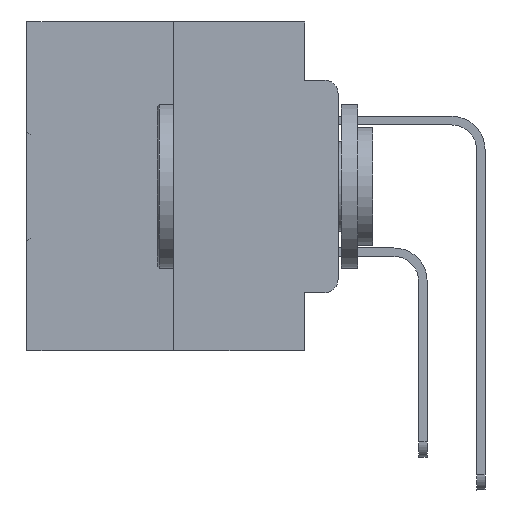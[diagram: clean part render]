
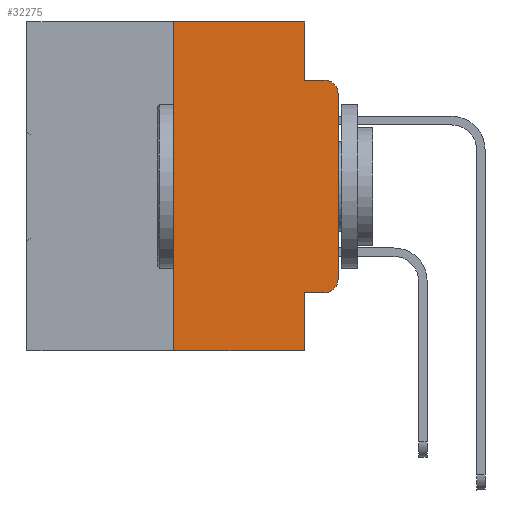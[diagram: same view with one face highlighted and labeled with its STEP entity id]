
A CAD part, left-side view. The second image highlights one B-rep face of the part: STEP entity #32275.
In plain terms, the highlighted planar face has unit normal (-1, 0, 0).
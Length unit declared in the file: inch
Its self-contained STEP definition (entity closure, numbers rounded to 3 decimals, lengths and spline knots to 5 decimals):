
#17 = ORIENTED_EDGE ( 'NONE', *, *, #22693, .F. ) ;
#160 = CARTESIAN_POINT ( 'NONE',  ( 0., 0.25, -0.5 ) ) ;
#294 = VERTEX_POINT ( 'NONE', #9027 ) ;
#494 = CARTESIAN_POINT ( 'NONE',  ( 0., 0.051, 0. ) ) ;
#1217 = VERTEX_POINT ( 'NONE', #7982 ) ;
#1354 = EDGE_LOOP ( 'NONE', ( #4849, #23765, #13144, #14403, #23952, #17, #20782, #31166, #22325, #22549 ) ) ;
#1962 = EDGE_CURVE ( 'NONE', #12531, #294, #4394, .T. ) ;
#2520 = DIRECTION ( 'NONE',  ( 0., 0., -1. ) ) ;
#3764 = DIRECTION ( 'NONE',  ( 0., -1., 0. ) ) ;
#4275 = AXIS2_PLACEMENT_3D ( 'NONE', #15778, #12622, #2520 ) ;
#4394 = LINE ( 'NONE', #23625, #15145 ) ;
#4592 = CARTESIAN_POINT ( 'NONE',  ( 0., 0.02, -0.1085 ) ) ;
#4849 = ORIENTED_EDGE ( 'NONE', *, *, #17953, .T. ) ;
#4910 = LINE ( 'NONE', #23252, #16567 ) ;
#6462 = VERTEX_POINT ( 'NONE', #9750 ) ;
#6599 = VERTEX_POINT ( 'NONE', #13415 ) ;
#6658 = LINE ( 'NONE', #19601, #23281 ) ;
#7982 = CARTESIAN_POINT ( 'NONE',  ( 0., 0.02, -0.0885 ) ) ;
#8341 = AXIS2_PLACEMENT_3D ( 'NONE', #23910, #29154, #18485 ) ;
#8583 = VERTEX_POINT ( 'NONE', #11410 ) ;
#8938 = DIRECTION ( 'NONE',  ( 0., 0., 1. ) ) ;
#9027 = CARTESIAN_POINT ( 'NONE',  ( 0., 0.051, -0.0885 ) ) ;
#9750 = CARTESIAN_POINT ( 'NONE',  ( 0., 0., -0.1085 ) ) ;
#10086 = EDGE_CURVE ( 'NONE', #6462, #1217, #32344, .T. ) ;
#10628 = VECTOR ( 'NONE', #26428, 39.37008 ) ;
#11410 = CARTESIAN_POINT ( 'NONE',  ( 0., 0.051, -0.4115 ) ) ;
#11671 = VECTOR ( 'NONE', #28363, 39.37008 ) ;
#11868 = VERTEX_POINT ( 'NONE', #20159 ) ;
#11936 = CARTESIAN_POINT ( 'NONE',  ( 0., 0., 0. ) ) ;
#12411 = DIRECTION ( 'NONE',  ( 0., 0., -1. ) ) ;
#12504 = VERTEX_POINT ( 'NONE', #160 ) ;
#12531 = VERTEX_POINT ( 'NONE', #494 ) ;
#12622 = DIRECTION ( 'NONE',  ( -1., 0., 0. ) ) ;
#13144 = ORIENTED_EDGE ( 'NONE', *, *, #33057, .F. ) ;
#13415 = CARTESIAN_POINT ( 'NONE',  ( 0., 0.25, 0. ) ) ;
#14403 = ORIENTED_EDGE ( 'NONE', *, *, #1962, .F. ) ;
#15058 = DIRECTION ( 'NONE',  ( 0., 0., 1. ) ) ;
#15145 = VECTOR ( 'NONE', #26060, 39.37008 ) ;
#15373 = CARTESIAN_POINT ( 'NONE',  ( 0., 0.473, -0.5 ) ) ;
#15761 = CARTESIAN_POINT ( 'NONE',  ( 0., 0.051, -0.0885 ) ) ;
#15778 = CARTESIAN_POINT ( 'NONE',  ( 0., 0.02, -0.3915 ) ) ;
#15942 = CARTESIAN_POINT ( 'NONE',  ( 0., 0.051, -0.5 ) ) ;
#16567 = VECTOR ( 'NONE', #12411, 39.37008 ) ;
#17953 = EDGE_CURVE ( 'NONE', #22711, #6462, #28353, .T. ) ;
#18129 = EDGE_CURVE ( 'NONE', #11868, #22711, #21593, .T. ) ;
#18485 = DIRECTION ( 'NONE',  ( 0., 0., -1. ) ) ;
#18568 = EDGE_CURVE ( 'NONE', #8583, #31263, #4910, .T. ) ;
#18815 = FACE_OUTER_BOUND ( 'NONE', #1354, .T. ) ;
#18874 = LINE ( 'NONE', #15373, #27511 ) ;
#19424 = CARTESIAN_POINT ( 'NONE',  ( 0., 0., -0.3915 ) ) ;
#19601 = CARTESIAN_POINT ( 'NONE',  ( 0., 0.25, 0. ) ) ;
#19784 = VECTOR ( 'NONE', #3764, 39.37008 ) ;
#20159 = CARTESIAN_POINT ( 'NONE',  ( 0., 0.02, -0.4115 ) ) ;
#20326 = LINE ( 'NONE', #28724, #11671 ) ;
#20782 = ORIENTED_EDGE ( 'NONE', *, *, #24681, .T. ) ;
#21019 = LINE ( 'NONE', #15761, #10628 ) ;
#21111 = PLANE ( 'NONE',  #8341 ) ;
#21593 = CIRCLE ( 'NONE', #4275, 0.02 ) ;
#22325 = ORIENTED_EDGE ( 'NONE', *, *, #32499, .T. ) ;
#22549 = ORIENTED_EDGE ( 'NONE', *, *, #18129, .T. ) ;
#22693 = EDGE_CURVE ( 'NONE', #12504, #6599, #6658, .T. ) ;
#22711 = VERTEX_POINT ( 'NONE', #19424 ) ;
#23252 = CARTESIAN_POINT ( 'NONE',  ( 0., 0.051, 0. ) ) ;
#23281 = VECTOR ( 'NONE', #8938, 39.37008 ) ;
#23625 = CARTESIAN_POINT ( 'NONE',  ( 0., 0.051, 0. ) ) ;
#23765 = ORIENTED_EDGE ( 'NONE', *, *, #10086, .T. ) ;
#23910 = CARTESIAN_POINT ( 'NONE',  ( 0., 0.473, 0. ) ) ;
#23952 = ORIENTED_EDGE ( 'NONE', *, *, #27161, .F. ) ;
#24681 = EDGE_CURVE ( 'NONE', #12504, #31263, #18874, .T. ) ;
#26051 = DIRECTION ( 'NONE',  ( 0., -1., 0. ) ) ;
#26060 = DIRECTION ( 'NONE',  ( 0., 0., -1. ) ) ;
#26185 = AXIS2_PLACEMENT_3D ( 'NONE', #4592, #31144, #27819 ) ;
#26428 = DIRECTION ( 'NONE',  ( 0., -1., 0. ) ) ;
#26591 = VECTOR ( 'NONE', #15058, 39.37008 ) ;
#27161 = EDGE_CURVE ( 'NONE', #6599, #12531, #32936, .T. ) ;
#27511 = VECTOR ( 'NONE', #26051, 39.37008 ) ;
#27679 = CARTESIAN_POINT ( 'NONE',  ( 0., 0.473, 0. ) ) ;
#27819 = DIRECTION ( 'NONE',  ( 0., 0., -1. ) ) ;
#28353 = LINE ( 'NONE', #11936, #26591 ) ;
#28363 = DIRECTION ( 'NONE',  ( 0., -1., 0. ) ) ;
#28724 = CARTESIAN_POINT ( 'NONE',  ( 0., 0.051, -0.4115 ) ) ;
#29154 = DIRECTION ( 'NONE',  ( 1., 0., 0. ) ) ;
#31144 = DIRECTION ( 'NONE',  ( -1., 0., 0. ) ) ;
#31166 = ORIENTED_EDGE ( 'NONE', *, *, #18568, .F. ) ;
#31263 = VERTEX_POINT ( 'NONE', #15942 ) ;
#32275 = ADVANCED_FACE ( 'NONE', ( #18815 ), #21111, .F. ) ;
#32344 = CIRCLE ( 'NONE', #26185, 0.02 ) ;
#32499 = EDGE_CURVE ( 'NONE', #8583, #11868, #20326, .T. ) ;
#32936 = LINE ( 'NONE', #27679, #19784 ) ;
#33057 = EDGE_CURVE ( 'NONE', #294, #1217, #21019, .T. ) ;
